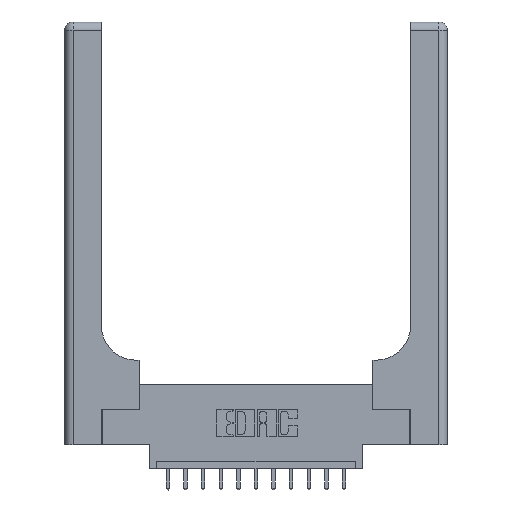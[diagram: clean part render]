
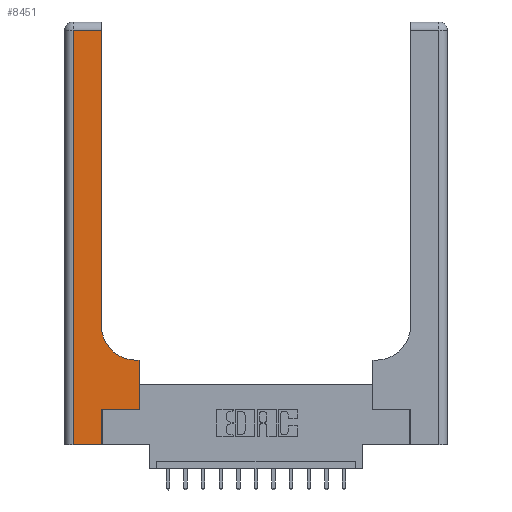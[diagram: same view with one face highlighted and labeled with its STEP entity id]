
A CAD part, top view. The second image highlights one B-rep face of the part: STEP entity #8451.
In plain terms, the highlighted planar face has unit normal (0, 0, 1).
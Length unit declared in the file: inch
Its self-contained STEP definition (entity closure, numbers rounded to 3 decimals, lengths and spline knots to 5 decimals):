
#17 = CARTESIAN_POINT ( 'NONE',  ( 0., 0., 0.37 ) ) ;
#248 = VERTEX_POINT ( 'NONE', #13676 ) ;
#254 = CARTESIAN_POINT ( 'NONE',  ( 0.26, 3., 0.37 ) ) ;
#388 = EDGE_CURVE ( 'NONE', #6112, #13205, #4518, .T. ) ;
#514 = EDGE_CURVE ( 'NONE', #16264, #4079, #14209, .T. ) ;
#564 = DIRECTION ( 'NONE',  ( 0., 1., 0. ) ) ;
#1472 = LINE ( 'NONE', #9265, #10777 ) ;
#1540 = VERTEX_POINT ( 'NONE', #4199 ) ;
#1758 = DIRECTION ( 'NONE',  ( 1., 0., 0. ) ) ;
#1786 = DIRECTION ( 'NONE',  ( 1., 0., 0. ) ) ;
#2241 = VERTEX_POINT ( 'NONE', #6709 ) ;
#2596 = CARTESIAN_POINT ( 'NONE',  ( 0., 2.94, 0.37 ) ) ;
#2613 = VECTOR ( 'NONE', #15196, 39.37008 ) ;
#2695 = ORIENTED_EDGE ( 'NONE', *, *, #7370, .T. ) ;
#3709 = ORIENTED_EDGE ( 'NONE', *, *, #9899, .T. ) ;
#3863 = ORIENTED_EDGE ( 'NONE', *, *, #12485, .T. ) ;
#4005 = EDGE_CURVE ( 'NONE', #4079, #7374, #1472, .T. ) ;
#4079 = VERTEX_POINT ( 'NONE', #10596 ) ;
#4199 = CARTESIAN_POINT ( 'NONE',  ( 0.26, 0.85, 0.37 ) ) ;
#4349 = CIRCLE ( 'NONE', #4429, 0.25 ) ;
#4429 = AXIS2_PLACEMENT_3D ( 'NONE', #14157, #14324, #1786 ) ;
#4518 = LINE ( 'NONE', #9871, #15968 ) ;
#4802 = PLANE ( 'NONE',  #8171 ) ;
#4994 = CARTESIAN_POINT ( 'NONE',  ( 0.26, 0.6, 0.37 ) ) ;
#6094 = VECTOR ( 'NONE', #14054, 39.37008 ) ;
#6112 = VERTEX_POINT ( 'NONE', #16121 ) ;
#6409 = VERTEX_POINT ( 'NONE', #12964 ) ;
#6709 = CARTESIAN_POINT ( 'NONE',  ( 0.26, 2.94, 0.37 ) ) ;
#6959 = EDGE_CURVE ( 'NONE', #7374, #6112, #8706, .T. ) ;
#6986 = EDGE_LOOP ( 'NONE', ( #12606, #3709, #10372, #8796, #14889, #8996, #11405, #3863, #2695 ) ) ;
#7370 = EDGE_CURVE ( 'NONE', #6409, #1540, #4349, .T. ) ;
#7374 = VERTEX_POINT ( 'NONE', #12982 ) ;
#7469 = FACE_OUTER_BOUND ( 'NONE', #6986, .T. ) ;
#8171 = AXIS2_PLACEMENT_3D ( 'NONE', #8733, #8623, #15017 ) ;
#8451 = ADVANCED_FACE ( 'NONE', ( #7469 ), #4802, .F. ) ;
#8538 = DIRECTION ( 'NONE',  ( 0., 1., 0. ) ) ;
#8623 = DIRECTION ( 'NONE',  ( 0., 0., -1. ) ) ;
#8706 = LINE ( 'NONE', #14303, #13483 ) ;
#8733 = CARTESIAN_POINT ( 'NONE',  ( 0., 3., 0.37 ) ) ;
#8796 = ORIENTED_EDGE ( 'NONE', *, *, #514, .T. ) ;
#8996 = ORIENTED_EDGE ( 'NONE', *, *, #6959, .T. ) ;
#9265 = CARTESIAN_POINT ( 'NONE',  ( 0.265, 0., 0.37 ) ) ;
#9459 = LINE ( 'NONE', #254, #12442 ) ;
#9871 = CARTESIAN_POINT ( 'NONE',  ( 0.528, 0.25, 0.37 ) ) ;
#9899 = EDGE_CURVE ( 'NONE', #2241, #248, #14892, .T. ) ;
#9972 = LINE ( 'NONE', #11911, #10955 ) ;
#10372 = ORIENTED_EDGE ( 'NONE', *, *, #11200, .T. ) ;
#10596 = CARTESIAN_POINT ( 'NONE',  ( 0.265, 0., 0.37 ) ) ;
#10777 = VECTOR ( 'NONE', #564, 39.37008 ) ;
#10955 = VECTOR ( 'NONE', #15820, 39.37008 ) ;
#11200 = EDGE_CURVE ( 'NONE', #248, #16264, #9972, .T. ) ;
#11405 = ORIENTED_EDGE ( 'NONE', *, *, #388, .T. ) ;
#11911 = CARTESIAN_POINT ( 'NONE',  ( 0.06, 3., 0.37 ) ) ;
#12313 = CARTESIAN_POINT ( 'NONE',  ( 0.528, 0.6, 0.37 ) ) ;
#12442 = VECTOR ( 'NONE', #8538, 39.37008 ) ;
#12485 = EDGE_CURVE ( 'NONE', #13205, #6409, #13691, .T. ) ;
#12606 = ORIENTED_EDGE ( 'NONE', *, *, #16085, .T. ) ;
#12808 = CARTESIAN_POINT ( 'NONE',  ( 0.06, 0., 0.37 ) ) ;
#12964 = CARTESIAN_POINT ( 'NONE',  ( 0.51, 0.6, 0.37 ) ) ;
#12982 = CARTESIAN_POINT ( 'NONE',  ( 0.265, 0.25, 0.37 ) ) ;
#13205 = VERTEX_POINT ( 'NONE', #12313 ) ;
#13483 = VECTOR ( 'NONE', #1758, 39.37008 ) ;
#13676 = CARTESIAN_POINT ( 'NONE',  ( 0.06, 2.94, 0.37 ) ) ;
#13691 = LINE ( 'NONE', #4994, #16032 ) ;
#14054 = DIRECTION ( 'NONE',  ( 1., 0., 0. ) ) ;
#14157 = CARTESIAN_POINT ( 'NONE',  ( 0.51, 0.85, 0.37 ) ) ;
#14209 = LINE ( 'NONE', #17, #6094 ) ;
#14303 = CARTESIAN_POINT ( 'NONE',  ( 0.265, 0.25, 0.37 ) ) ;
#14324 = DIRECTION ( 'NONE',  ( 0., 0., -1. ) ) ;
#14889 = ORIENTED_EDGE ( 'NONE', *, *, #4005, .T. ) ;
#14892 = LINE ( 'NONE', #2596, #2613 ) ;
#14991 = DIRECTION ( 'NONE',  ( -1., 0., 0. ) ) ;
#15017 = DIRECTION ( 'NONE',  ( -1., 0., 0. ) ) ;
#15030 = DIRECTION ( 'NONE',  ( 0., 1., 0. ) ) ;
#15196 = DIRECTION ( 'NONE',  ( -1., 0., 0. ) ) ;
#15820 = DIRECTION ( 'NONE',  ( 0., -1., 0. ) ) ;
#15968 = VECTOR ( 'NONE', #15030, 39.37008 ) ;
#16032 = VECTOR ( 'NONE', #14991, 39.37008 ) ;
#16085 = EDGE_CURVE ( 'NONE', #1540, #2241, #9459, .T. ) ;
#16121 = CARTESIAN_POINT ( 'NONE',  ( 0.528, 0.25, 0.37 ) ) ;
#16264 = VERTEX_POINT ( 'NONE', #12808 ) ;
